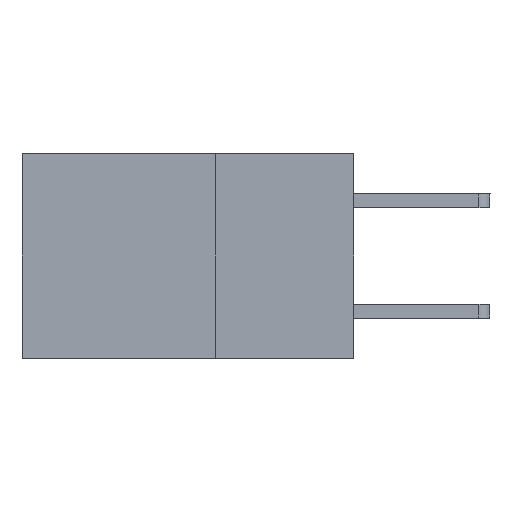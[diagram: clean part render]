
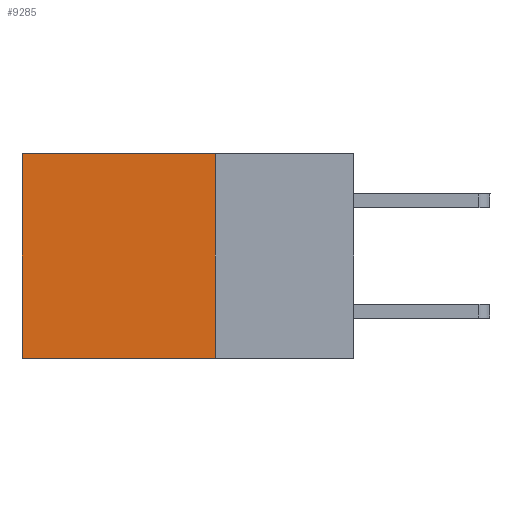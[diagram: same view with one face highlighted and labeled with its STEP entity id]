
A CAD part, left-side view. The second image highlights one B-rep face of the part: STEP entity #9285.
In plain terms, the highlighted planar face has unit normal (-1, 0, 0).
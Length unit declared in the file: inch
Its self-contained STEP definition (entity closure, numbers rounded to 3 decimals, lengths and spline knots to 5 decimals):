
#1399 = VERTEX_POINT ( 'NONE', #4361 ) ;
#1411 = VECTOR ( 'NONE', #7667, 39.37008 ) ;
#2100 = DIRECTION ( 'NONE',  ( 0., 0., -1. ) ) ;
#2315 = CARTESIAN_POINT ( 'NONE',  ( 0.2875, 0.25, 0. ) ) ;
#2989 = CARTESIAN_POINT ( 'NONE',  ( 0.2875, 0.25, 0. ) ) ;
#3031 = ORIENTED_EDGE ( 'NONE', *, *, #7162, .T. ) ;
#3044 = ORIENTED_EDGE ( 'NONE', *, *, #3373, .F. ) ;
#3053 = ORIENTED_EDGE ( 'NONE', *, *, #3153, .F. ) ;
#3056 = ORIENTED_EDGE ( 'NONE', *, *, #8842, .T. ) ;
#3092 = VECTOR ( 'NONE', #10895, 39.37008 ) ;
#3153 = EDGE_CURVE ( 'NONE', #7520, #1399, #10228, .T. ) ;
#3373 = EDGE_CURVE ( 'NONE', #1399, #6288, #4092, .T. ) ;
#3812 = VECTOR ( 'NONE', #9501, 39.37008 ) ;
#3938 = LINE ( 'NONE', #9943, #8553 ) ;
#4092 = LINE ( 'NONE', #8677, #3812 ) ;
#4361 = CARTESIAN_POINT ( 'NONE',  ( 0.2875, 0.25, -0.37 ) ) ;
#5711 = PLANE ( 'NONE',  #7705 ) ;
#5814 = EDGE_LOOP ( 'NONE', ( #3031, #3044, #3053, #3056 ) ) ;
#6288 = VERTEX_POINT ( 'NONE', #7116 ) ;
#7116 = CARTESIAN_POINT ( 'NONE',  ( 0.2875, 0.6, -0.37 ) ) ;
#7162 = EDGE_CURVE ( 'NONE', #10697, #6288, #3938, .T. ) ;
#7469 = DIRECTION ( 'NONE',  ( 1., 0., 0. ) ) ;
#7520 = VERTEX_POINT ( 'NONE', #8134 ) ;
#7667 = DIRECTION ( 'NONE',  ( 0., 1., 0. ) ) ;
#7705 = AXIS2_PLACEMENT_3D ( 'NONE', #2989, #7469, #2100 ) ;
#7783 = CARTESIAN_POINT ( 'NONE',  ( 0.2875, 0.6, 0. ) ) ;
#8134 = CARTESIAN_POINT ( 'NONE',  ( 0.2875, 0.25, 0. ) ) ;
#8553 = VECTOR ( 'NONE', #10750, 39.37008 ) ;
#8677 = CARTESIAN_POINT ( 'NONE',  ( 0.2875, 0.25, -0.37 ) ) ;
#8842 = EDGE_CURVE ( 'NONE', #7520, #10697, #10906, .T. ) ;
#9285 = ADVANCED_FACE ( 'NONE', ( #10157 ), #5711, .F. ) ;
#9501 = DIRECTION ( 'NONE',  ( 0., 1., 0. ) ) ;
#9943 = CARTESIAN_POINT ( 'NONE',  ( 0.2875, 0.6, 0. ) ) ;
#10104 = CARTESIAN_POINT ( 'NONE',  ( 0.2875, 0.25, 0. ) ) ;
#10157 = FACE_OUTER_BOUND ( 'NONE', #5814, .T. ) ;
#10228 = LINE ( 'NONE', #10104, #3092 ) ;
#10697 = VERTEX_POINT ( 'NONE', #7783 ) ;
#10750 = DIRECTION ( 'NONE',  ( 0., 0., -1. ) ) ;
#10895 = DIRECTION ( 'NONE',  ( 0., 0., -1. ) ) ;
#10906 = LINE ( 'NONE', #2315, #1411 ) ;
